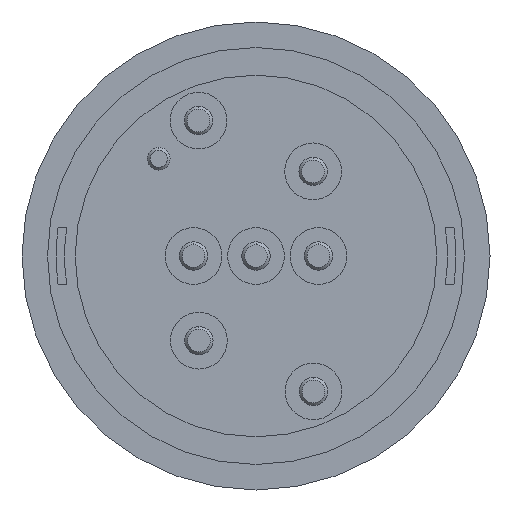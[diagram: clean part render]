
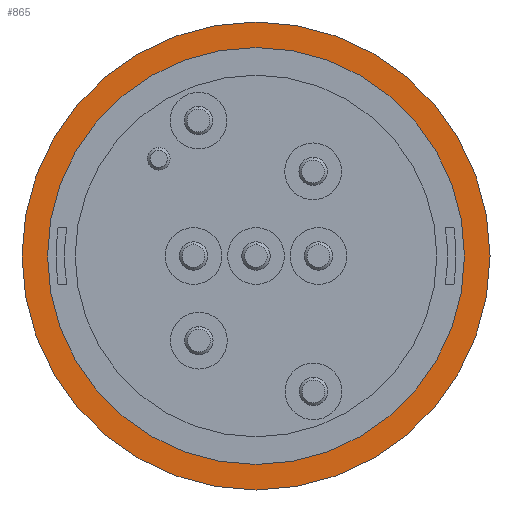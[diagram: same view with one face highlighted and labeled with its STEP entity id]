
A CAD part, front view. The second image highlights one B-rep face of the part: STEP entity #865.
In plain terms, the highlighted planar face has unit normal (0, -1, 0).
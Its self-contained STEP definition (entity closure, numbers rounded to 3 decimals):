
#61 = CIRCLE ( 'NONE', #5395, 8.25 ) ;
#144 = ORIENTED_EDGE ( 'NONE', *, *, #597, .T. ) ;
#328 = DIRECTION ( 'NONE',  ( 0., 0., -1. ) ) ;
#367 = EDGE_CURVE ( 'NONE', #4166, #734, #6143, .T. ) ;
#597 = EDGE_CURVE ( 'NONE', #734, #4166, #61, .T. ) ;
#634 = DIRECTION ( 'NONE',  ( 0., 0., -1. ) ) ;
#734 = VERTEX_POINT ( 'NONE', #2861 ) ;
#865 = ADVANCED_FACE ( 'NONE', ( #4183, #5609 ), #4151, .T. ) ;
#972 = DIRECTION ( 'NONE',  ( 0., 0., -1. ) ) ;
#1137 = AXIS2_PLACEMENT_3D ( 'NONE', #6296, #5201, #972 ) ;
#1645 = CARTESIAN_POINT ( 'NONE',  ( 0., -3., 0. ) ) ;
#1731 = CARTESIAN_POINT ( 'NONE',  ( 0., -3., 0. ) ) ;
#2214 = CIRCLE ( 'NONE', #5754, 7.35 ) ;
#2461 = CIRCLE ( 'NONE', #1137, 7.35 ) ;
#2761 = EDGE_CURVE ( 'NONE', #3235, #4392, #2214, .T. ) ;
#2861 = CARTESIAN_POINT ( 'NONE',  ( 0., -3., 8.25 ) ) ;
#3067 = DIRECTION ( 'NONE',  ( 0., -1., 0. ) ) ;
#3235 = VERTEX_POINT ( 'NONE', #3506 ) ;
#3384 = AXIS2_PLACEMENT_3D ( 'NONE', #1731, #6104, #5153 ) ;
#3506 = CARTESIAN_POINT ( 'NONE',  ( 0., -3., 7.35 ) ) ;
#3518 = CARTESIAN_POINT ( 'NONE',  ( 0., -3., 0. ) ) ;
#3556 = EDGE_LOOP ( 'NONE', ( #144, #4009 ) ) ;
#3784 = CARTESIAN_POINT ( 'NONE',  ( 0., -3., 0. ) ) ;
#4009 = ORIENTED_EDGE ( 'NONE', *, *, #367, .T. ) ;
#4151 = PLANE ( 'NONE',  #3384 ) ;
#4166 = VERTEX_POINT ( 'NONE', #4578 ) ;
#4183 = FACE_BOUND ( 'NONE', #5706, .T. ) ;
#4280 = CARTESIAN_POINT ( 'NONE',  ( 0., -3., -7.35 ) ) ;
#4392 = VERTEX_POINT ( 'NONE', #4280 ) ;
#4459 = DIRECTION ( 'NONE',  ( 0., 0., -1. ) ) ;
#4578 = CARTESIAN_POINT ( 'NONE',  ( 0., -3., -8.25 ) ) ;
#4699 = EDGE_CURVE ( 'NONE', #4392, #3235, #2461, .T. ) ;
#4738 = DIRECTION ( 'NONE',  ( 0., -1., 0. ) ) ;
#4992 = AXIS2_PLACEMENT_3D ( 'NONE', #3518, #5469, #4459 ) ;
#5128 = ORIENTED_EDGE ( 'NONE', *, *, #4699, .F. ) ;
#5153 = DIRECTION ( 'NONE',  ( 0., 0., -1. ) ) ;
#5201 = DIRECTION ( 'NONE',  ( 0., -1., 0. ) ) ;
#5395 = AXIS2_PLACEMENT_3D ( 'NONE', #1645, #3067, #634 ) ;
#5469 = DIRECTION ( 'NONE',  ( 0., -1., 0. ) ) ;
#5609 = FACE_OUTER_BOUND ( 'NONE', #3556, .T. ) ;
#5706 = EDGE_LOOP ( 'NONE', ( #6259, #5128 ) ) ;
#5754 = AXIS2_PLACEMENT_3D ( 'NONE', #3784, #4738, #328 ) ;
#6104 = DIRECTION ( 'NONE',  ( 0., -1., 0. ) ) ;
#6143 = CIRCLE ( 'NONE', #4992, 8.25 ) ;
#6259 = ORIENTED_EDGE ( 'NONE', *, *, #2761, .F. ) ;
#6296 = CARTESIAN_POINT ( 'NONE',  ( 0., -3., 0. ) ) ;
